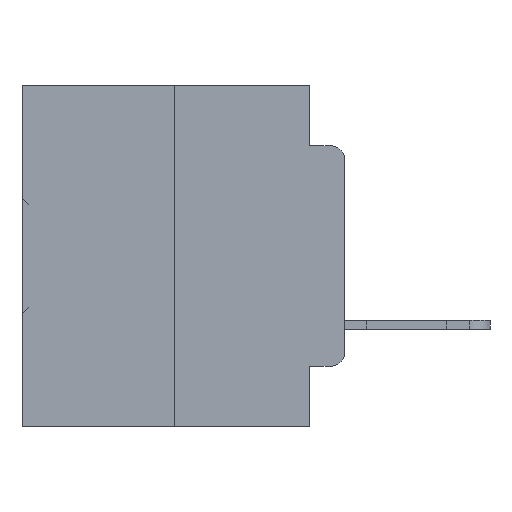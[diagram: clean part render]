
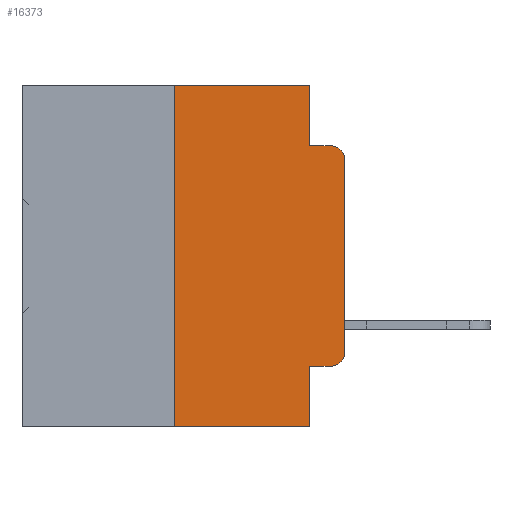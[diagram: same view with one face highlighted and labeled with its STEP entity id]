
A CAD part, left-side view. The second image highlights one B-rep face of the part: STEP entity #16373.
In plain terms, the highlighted planar face has unit normal (-1, 0, 0).
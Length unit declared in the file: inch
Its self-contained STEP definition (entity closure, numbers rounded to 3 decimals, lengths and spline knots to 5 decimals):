
#382 = ORIENTED_EDGE ( 'NONE', *, *, #11945, .F. ) ;
#806 = CARTESIAN_POINT ( 'NONE',  ( 0., 0.02, -0.0885 ) ) ;
#1117 = CARTESIAN_POINT ( 'NONE',  ( 0., 0.051, -0.4115 ) ) ;
#1622 = VECTOR ( 'NONE', #13235, 39.37008 ) ;
#2336 = VERTEX_POINT ( 'NONE', #24329 ) ;
#3189 = CARTESIAN_POINT ( 'NONE',  ( 0., 0.051, -0.0885 ) ) ;
#5984 = CARTESIAN_POINT ( 'NONE',  ( 0., 0.02, -0.4115 ) ) ;
#6399 = VECTOR ( 'NONE', #23371, 39.37008 ) ;
#7505 = CARTESIAN_POINT ( 'NONE',  ( 0., 0.25, 0. ) ) ;
#7683 = FACE_OUTER_BOUND ( 'NONE', #21492, .T. ) ;
#7735 = CARTESIAN_POINT ( 'NONE',  ( 0., 0., -0.3915 ) ) ;
#8039 = ORIENTED_EDGE ( 'NONE', *, *, #9924, .T. ) ;
#9141 = EDGE_CURVE ( 'NONE', #11390, #26151, #35711, .T. ) ;
#9203 = VECTOR ( 'NONE', #15459, 39.37008 ) ;
#9580 = AXIS2_PLACEMENT_3D ( 'NONE', #32012, #31875, #31487 ) ;
#9924 = EDGE_CURVE ( 'NONE', #33573, #27211, #25033, .T. ) ;
#10203 = DIRECTION ( 'NONE',  ( -1., 0., 0. ) ) ;
#10467 = CARTESIAN_POINT ( 'NONE',  ( 0., 0.02, -0.3915 ) ) ;
#10506 = DIRECTION ( 'NONE',  ( 0., 0., -1. ) ) ;
#11390 = VERTEX_POINT ( 'NONE', #14975 ) ;
#11753 = LINE ( 'NONE', #25615, #33371 ) ;
#11945 = EDGE_CURVE ( 'NONE', #33573, #25313, #29887, .T. ) ;
#11996 = VERTEX_POINT ( 'NONE', #28742 ) ;
#12063 = CARTESIAN_POINT ( 'NONE',  ( 0., 0.051, -0.5 ) ) ;
#12293 = VECTOR ( 'NONE', #33952, 39.37008 ) ;
#12780 = AXIS2_PLACEMENT_3D ( 'NONE', #10467, #10203, #10506 ) ;
#13235 = DIRECTION ( 'NONE',  ( 0., 0., -1. ) ) ;
#13756 = EDGE_CURVE ( 'NONE', #2336, #25313, #11753, .T. ) ;
#14065 = VECTOR ( 'NONE', #36036, 39.37008 ) ;
#14975 = CARTESIAN_POINT ( 'NONE',  ( 0., 0., -0.1085 ) ) ;
#15100 = EDGE_CURVE ( 'NONE', #17275, #11390, #29211, .T. ) ;
#15459 = DIRECTION ( 'NONE',  ( 0., -1., 0. ) ) ;
#15500 = CARTESIAN_POINT ( 'NONE',  ( 0., 0.051, -0.4115 ) ) ;
#16373 = ADVANCED_FACE ( 'NONE', ( #7683 ), #25900, .F. ) ;
#16544 = ORIENTED_EDGE ( 'NONE', *, *, #23130, .F. ) ;
#16996 = ORIENTED_EDGE ( 'NONE', *, *, #19773, .F. ) ;
#17275 = VERTEX_POINT ( 'NONE', #7735 ) ;
#17384 = VERTEX_POINT ( 'NONE', #34695 ) ;
#17434 = ORIENTED_EDGE ( 'NONE', *, *, #21352, .F. ) ;
#18584 = EDGE_CURVE ( 'NONE', #27211, #17275, #29082, .T. ) ;
#19773 = EDGE_CURVE ( 'NONE', #11996, #17384, #33842, .T. ) ;
#21352 = EDGE_CURVE ( 'NONE', #2336, #11996, #35404, .T. ) ;
#21492 = EDGE_LOOP ( 'NONE', ( #33200, #26697, #35657, #16544, #16996, #17434, #28583, #382, #8039, #22817 ) ) ;
#22163 = VECTOR ( 'NONE', #32758, 39.37008 ) ;
#22817 = ORIENTED_EDGE ( 'NONE', *, *, #18584, .T. ) ;
#22839 = VECTOR ( 'NONE', #31042, 39.37008 ) ;
#23073 = VERTEX_POINT ( 'NONE', #31944 ) ;
#23130 = EDGE_CURVE ( 'NONE', #17384, #23073, #32442, .T. ) ;
#23371 = DIRECTION ( 'NONE',  ( 0., -1., 0. ) ) ;
#24201 = CARTESIAN_POINT ( 'NONE',  ( 0., 0.051, 0. ) ) ;
#24329 = CARTESIAN_POINT ( 'NONE',  ( 0., 0.25, -0.5 ) ) ;
#25033 = LINE ( 'NONE', #15500, #9203 ) ;
#25313 = VERTEX_POINT ( 'NONE', #12063 ) ;
#25387 = DIRECTION ( 'NONE',  ( 0., 0., -1. ) ) ;
#25615 = CARTESIAN_POINT ( 'NONE',  ( 0., 0.473, -0.5 ) ) ;
#25650 = CARTESIAN_POINT ( 'NONE',  ( 0., 0.473, 0. ) ) ;
#25656 = DIRECTION ( 'NONE',  ( 0., -1., 0. ) ) ;
#25900 = PLANE ( 'NONE',  #30326 ) ;
#26151 = VERTEX_POINT ( 'NONE', #806 ) ;
#26389 = DIRECTION ( 'NONE',  ( 1., 0., 0. ) ) ;
#26697 = ORIENTED_EDGE ( 'NONE', *, *, #9141, .T. ) ;
#27211 = VERTEX_POINT ( 'NONE', #5984 ) ;
#28028 = LINE ( 'NONE', #3189, #6399 ) ;
#28583 = ORIENTED_EDGE ( 'NONE', *, *, #13756, .T. ) ;
#28742 = CARTESIAN_POINT ( 'NONE',  ( 0., 0.25, 0. ) ) ;
#29082 = CIRCLE ( 'NONE', #12780, 0.02 ) ;
#29211 = LINE ( 'NONE', #31887, #22163 ) ;
#29887 = LINE ( 'NONE', #31297, #22839 ) ;
#30264 = EDGE_CURVE ( 'NONE', #23073, #26151, #28028, .T. ) ;
#30326 = AXIS2_PLACEMENT_3D ( 'NONE', #25650, #26389, #25387 ) ;
#31042 = DIRECTION ( 'NONE',  ( 0., 0., -1. ) ) ;
#31297 = CARTESIAN_POINT ( 'NONE',  ( 0., 0.051, 0. ) ) ;
#31487 = DIRECTION ( 'NONE',  ( 0., 0., -1. ) ) ;
#31875 = DIRECTION ( 'NONE',  ( -1., 0., 0. ) ) ;
#31887 = CARTESIAN_POINT ( 'NONE',  ( 0., 0., 0. ) ) ;
#31944 = CARTESIAN_POINT ( 'NONE',  ( 0., 0.051, -0.0885 ) ) ;
#32012 = CARTESIAN_POINT ( 'NONE',  ( 0., 0.02, -0.1085 ) ) ;
#32442 = LINE ( 'NONE', #24201, #1622 ) ;
#32758 = DIRECTION ( 'NONE',  ( 0., 0., 1. ) ) ;
#33200 = ORIENTED_EDGE ( 'NONE', *, *, #15100, .T. ) ;
#33371 = VECTOR ( 'NONE', #25656, 39.37008 ) ;
#33573 = VERTEX_POINT ( 'NONE', #1117 ) ;
#33842 = LINE ( 'NONE', #35160, #12293 ) ;
#33952 = DIRECTION ( 'NONE',  ( 0., -1., 0. ) ) ;
#34695 = CARTESIAN_POINT ( 'NONE',  ( 0., 0.051, 0. ) ) ;
#35160 = CARTESIAN_POINT ( 'NONE',  ( 0., 0.473, 0. ) ) ;
#35404 = LINE ( 'NONE', #7505, #14065 ) ;
#35657 = ORIENTED_EDGE ( 'NONE', *, *, #30264, .F. ) ;
#35711 = CIRCLE ( 'NONE', #9580, 0.02 ) ;
#36036 = DIRECTION ( 'NONE',  ( 0., 0., 1. ) ) ;
